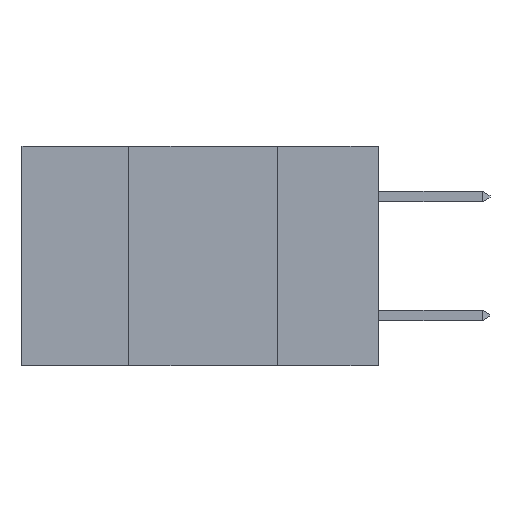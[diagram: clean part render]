
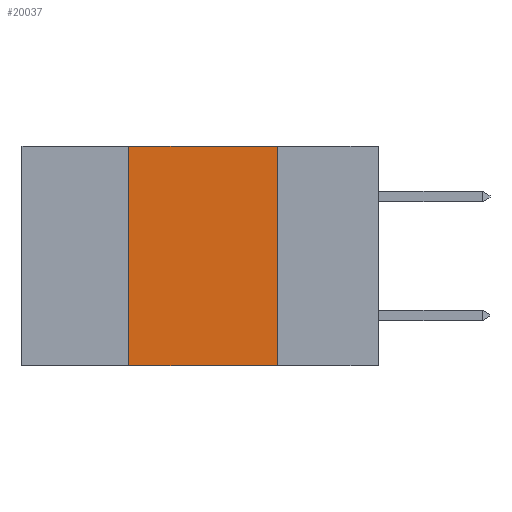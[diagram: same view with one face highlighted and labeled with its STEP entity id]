
A CAD part, left-side view. The second image highlights one B-rep face of the part: STEP entity #20037.
In plain terms, the highlighted planar face has unit normal (-1, 0, 0).
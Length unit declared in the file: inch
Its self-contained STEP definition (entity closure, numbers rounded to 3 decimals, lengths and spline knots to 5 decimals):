
#303 = CARTESIAN_POINT ( 'NONE',  ( 0., 0.17, 0. ) ) ;
#1126 = ORIENTED_EDGE ( 'NONE', *, *, #8281, .F. ) ;
#1774 = EDGE_CURVE ( 'NONE', #11408, #26152, #4092, .T. ) ;
#2725 = DIRECTION ( 'NONE',  ( 0., 0., -1. ) ) ;
#3473 = ORIENTED_EDGE ( 'NONE', *, *, #16005, .F. ) ;
#3893 = VECTOR ( 'NONE', #2725, 39.37008 ) ;
#4092 = LINE ( 'NONE', #12153, #9797 ) ;
#4790 = PLANE ( 'NONE',  #28429 ) ;
#5649 = DIRECTION ( 'NONE',  ( 0., 0., 1. ) ) ;
#6420 = LINE ( 'NONE', #8811, #18495 ) ;
#6957 = VERTEX_POINT ( 'NONE', #21606 ) ;
#7147 = CARTESIAN_POINT ( 'NONE',  ( 0., 0.6, 0. ) ) ;
#7244 = DIRECTION ( 'NONE',  ( 0., 0., -1. ) ) ;
#7560 = CARTESIAN_POINT ( 'NONE',  ( 0., 0.6, -0.37 ) ) ;
#7602 = EDGE_CURVE ( 'NONE', #11408, #18533, #17937, .T. ) ;
#8281 = EDGE_CURVE ( 'NONE', #6957, #18533, #10360, .T. ) ;
#8811 = CARTESIAN_POINT ( 'NONE',  ( 0., 0.6, 0. ) ) ;
#9797 = VECTOR ( 'NONE', #5649, 39.37008 ) ;
#10328 = ORIENTED_EDGE ( 'NONE', *, *, #7602, .T. ) ;
#10360 = LINE ( 'NONE', #303, #3893 ) ;
#10776 = FACE_OUTER_BOUND ( 'NONE', #25006, .T. ) ;
#11408 = VERTEX_POINT ( 'NONE', #23585 ) ;
#12153 = CARTESIAN_POINT ( 'NONE',  ( 0., 0.42, 0. ) ) ;
#13364 = CARTESIAN_POINT ( 'NONE',  ( 0., 0.42, 0. ) ) ;
#14168 = ORIENTED_EDGE ( 'NONE', *, *, #1774, .F. ) ;
#16005 = EDGE_CURVE ( 'NONE', #26152, #6957, #6420, .T. ) ;
#17937 = LINE ( 'NONE', #7560, #29668 ) ;
#18495 = VECTOR ( 'NONE', #23123, 39.37008 ) ;
#18533 = VERTEX_POINT ( 'NONE', #29814 ) ;
#20037 = ADVANCED_FACE ( 'NONE', ( #10776 ), #4790, .F. ) ;
#21600 = DIRECTION ( 'NONE',  ( 1., 0., 0. ) ) ;
#21606 = CARTESIAN_POINT ( 'NONE',  ( 0., 0.17, 0. ) ) ;
#23123 = DIRECTION ( 'NONE',  ( 0., -1., 0. ) ) ;
#23585 = CARTESIAN_POINT ( 'NONE',  ( 0., 0.42, -0.37 ) ) ;
#24256 = DIRECTION ( 'NONE',  ( 0., -1., 0. ) ) ;
#25006 = EDGE_LOOP ( 'NONE', ( #1126, #3473, #14168, #10328 ) ) ;
#26152 = VERTEX_POINT ( 'NONE', #13364 ) ;
#28429 = AXIS2_PLACEMENT_3D ( 'NONE', #7147, #21600, #7244 ) ;
#29668 = VECTOR ( 'NONE', #24256, 39.37008 ) ;
#29814 = CARTESIAN_POINT ( 'NONE',  ( 0., 0.17, -0.37 ) ) ;
